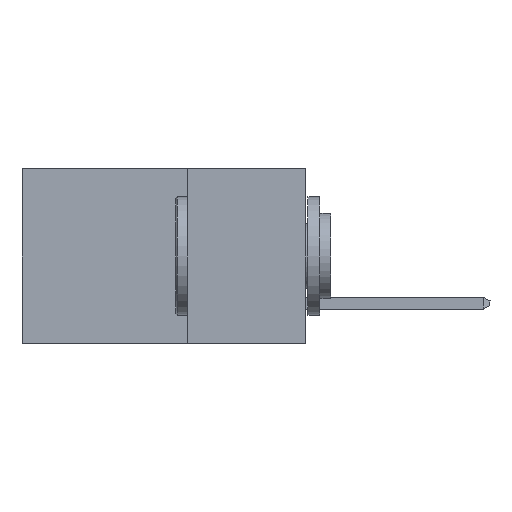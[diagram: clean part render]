
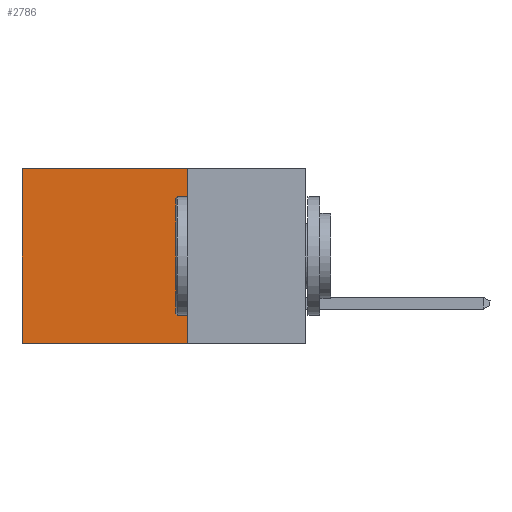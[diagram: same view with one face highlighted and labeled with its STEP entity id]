
A CAD part, left-side view. The second image highlights one B-rep face of the part: STEP entity #2786.
In plain terms, the highlighted planar face has unit normal (-1, 0, 0).
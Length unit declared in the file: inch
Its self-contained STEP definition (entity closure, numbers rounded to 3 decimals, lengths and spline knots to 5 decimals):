
#237 = DIRECTION ( 'NONE',  ( 1., 0., 0. ) ) ;
#871 = DIRECTION ( 'NONE',  ( 0., 1., 0. ) ) ;
#1740 = CARTESIAN_POINT ( 'NONE',  ( 0.2615, 0.25, -0.37 ) ) ;
#1887 = DIRECTION ( 'NONE',  ( 0., 1., 0. ) ) ;
#2075 = CARTESIAN_POINT ( 'NONE',  ( 0.2615, 0.6, 0. ) ) ;
#2077 = ORIENTED_EDGE ( 'NONE', *, *, #16278, .F. ) ;
#2691 = CARTESIAN_POINT ( 'NONE',  ( 0.2615, 0.25, -0.37 ) ) ;
#2786 = ADVANCED_FACE ( 'NONE', ( #10354 ), #10440, .F. ) ;
#2825 = EDGE_CURVE ( 'NONE', #5598, #16037, #3280, .T. ) ;
#3280 = LINE ( 'NONE', #8885, #6619 ) ;
#4124 = CARTESIAN_POINT ( 'NONE',  ( 0.2615, 0.25, 0. ) ) ;
#5231 = VECTOR ( 'NONE', #5448, 39.37008 ) ;
#5448 = DIRECTION ( 'NONE',  ( 0., 0., -1. ) ) ;
#5598 = VERTEX_POINT ( 'NONE', #4124 ) ;
#5866 = VECTOR ( 'NONE', #9672, 39.37008 ) ;
#6242 = EDGE_CURVE ( 'NONE', #16037, #8108, #13793, .T. ) ;
#6599 = AXIS2_PLACEMENT_3D ( 'NONE', #12928, #237, #11561 ) ;
#6619 = VECTOR ( 'NONE', #1887, 39.37008 ) ;
#7365 = ORIENTED_EDGE ( 'NONE', *, *, #7614, .F. ) ;
#7614 = EDGE_CURVE ( 'NONE', #5598, #14198, #18022, .T. ) ;
#7874 = LINE ( 'NONE', #13463, #12908 ) ;
#8108 = VERTEX_POINT ( 'NONE', #12952 ) ;
#8885 = CARTESIAN_POINT ( 'NONE',  ( 0.2615, 0.25, 0. ) ) ;
#9672 = DIRECTION ( 'NONE',  ( 0., 0., -1. ) ) ;
#10354 = FACE_OUTER_BOUND ( 'NONE', #11834, .T. ) ;
#10440 = PLANE ( 'NONE',  #6599 ) ;
#11561 = DIRECTION ( 'NONE',  ( 0., 0., -1. ) ) ;
#11834 = EDGE_LOOP ( 'NONE', ( #12671, #2077, #7365, #16779 ) ) ;
#12671 = ORIENTED_EDGE ( 'NONE', *, *, #6242, .T. ) ;
#12908 = VECTOR ( 'NONE', #871, 39.37008 ) ;
#12928 = CARTESIAN_POINT ( 'NONE',  ( 0.2615, 0.25, -0.37 ) ) ;
#12952 = CARTESIAN_POINT ( 'NONE',  ( 0.2615, 0.6, -0.37 ) ) ;
#13463 = CARTESIAN_POINT ( 'NONE',  ( 0.2615, 0.25, -0.37 ) ) ;
#13793 = LINE ( 'NONE', #16641, #5866 ) ;
#14198 = VERTEX_POINT ( 'NONE', #1740 ) ;
#16037 = VERTEX_POINT ( 'NONE', #2075 ) ;
#16278 = EDGE_CURVE ( 'NONE', #14198, #8108, #7874, .T. ) ;
#16641 = CARTESIAN_POINT ( 'NONE',  ( 0.2615, 0.6, -0.37 ) ) ;
#16779 = ORIENTED_EDGE ( 'NONE', *, *, #2825, .T. ) ;
#18022 = LINE ( 'NONE', #2691, #5231 ) ;
